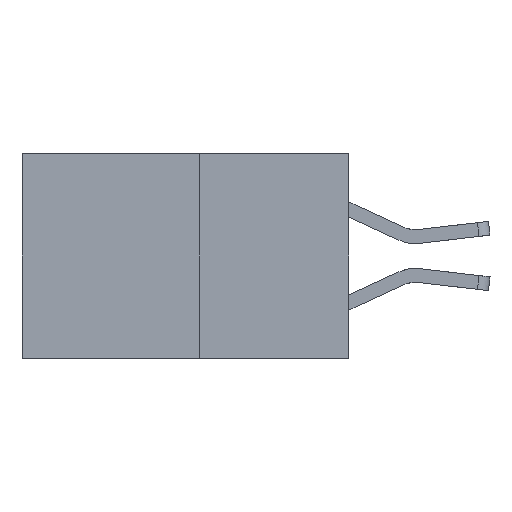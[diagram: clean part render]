
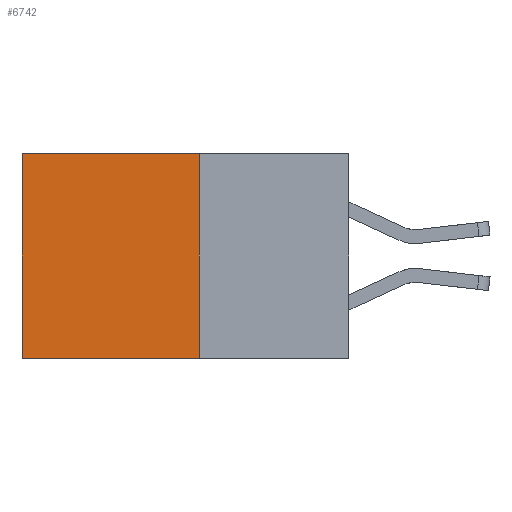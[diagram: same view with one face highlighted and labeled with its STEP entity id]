
A CAD part, left-side view. The second image highlights one B-rep face of the part: STEP entity #6742.
In plain terms, the highlighted planar face has unit normal (-1, 0, 0).
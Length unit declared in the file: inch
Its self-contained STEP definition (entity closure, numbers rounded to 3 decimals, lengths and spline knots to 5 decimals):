
#52 = ORIENTED_EDGE ( 'NONE', *, *, #1858, .T. ) ;
#1047 = VECTOR ( 'NONE', #1364, 39.37008 ) ;
#1349 = LINE ( 'NONE', #10455, #1047 ) ;
#1364 = DIRECTION ( 'NONE',  ( 0., 1., 0. ) ) ;
#1858 = EDGE_CURVE ( 'NONE', #4955, #6531, #1982, .T. ) ;
#1945 = LINE ( 'NONE', #10890, #11293 ) ;
#1982 = LINE ( 'NONE', #11210, #6603 ) ;
#2382 = ORIENTED_EDGE ( 'NONE', *, *, #6188, .F. ) ;
#2628 = PLANE ( 'NONE',  #7775 ) ;
#3532 = CARTESIAN_POINT ( 'NONE',  ( 0.277, 0.59, -0.37 ) ) ;
#3776 = VERTEX_POINT ( 'NONE', #3532 ) ;
#4144 = CARTESIAN_POINT ( 'NONE',  ( 0.277, 0.59, 0. ) ) ;
#4489 = CARTESIAN_POINT ( 'NONE',  ( 0.277, 0.27, -0.37 ) ) ;
#4505 = EDGE_CURVE ( 'NONE', #6531, #3776, #9742, .T. ) ;
#4569 = ORIENTED_EDGE ( 'NONE', *, *, #5871, .F. ) ;
#4955 = VERTEX_POINT ( 'NONE', #5926 ) ;
#5400 = DIRECTION ( 'NONE',  ( 1., 0., 0. ) ) ;
#5871 = EDGE_CURVE ( 'NONE', #10681, #3776, #1349, .T. ) ;
#5926 = CARTESIAN_POINT ( 'NONE',  ( 0.277, 0.27, 0. ) ) ;
#6188 = EDGE_CURVE ( 'NONE', #4955, #10681, #1945, .T. ) ;
#6531 = VERTEX_POINT ( 'NONE', #4144 ) ;
#6603 = VECTOR ( 'NONE', #11321, 39.37008 ) ;
#6690 = ORIENTED_EDGE ( 'NONE', *, *, #4505, .T. ) ;
#6742 = ADVANCED_FACE ( 'NONE', ( #9196 ), #2628, .F. ) ;
#6964 = CARTESIAN_POINT ( 'NONE',  ( 0.277, 0.27, -0.37 ) ) ;
#7775 = AXIS2_PLACEMENT_3D ( 'NONE', #4489, #5400, #11611 ) ;
#8327 = DIRECTION ( 'NONE',  ( 0., 0., -1. ) ) ;
#9196 = FACE_OUTER_BOUND ( 'NONE', #10832, .T. ) ;
#9742 = LINE ( 'NONE', #11450, #11726 ) ;
#10455 = CARTESIAN_POINT ( 'NONE',  ( 0.277, 0.27, -0.37 ) ) ;
#10681 = VERTEX_POINT ( 'NONE', #6964 ) ;
#10832 = EDGE_LOOP ( 'NONE', ( #6690, #4569, #2382, #52 ) ) ;
#10890 = CARTESIAN_POINT ( 'NONE',  ( 0.277, 0.27, -0.37 ) ) ;
#11210 = CARTESIAN_POINT ( 'NONE',  ( 0.277, 0.27, 0. ) ) ;
#11293 = VECTOR ( 'NONE', #8327, 39.37008 ) ;
#11321 = DIRECTION ( 'NONE',  ( 0., 1., 0. ) ) ;
#11450 = CARTESIAN_POINT ( 'NONE',  ( 0.277, 0.59, -0.37 ) ) ;
#11557 = DIRECTION ( 'NONE',  ( 0., 0., -1. ) ) ;
#11611 = DIRECTION ( 'NONE',  ( 0., 0., -1. ) ) ;
#11726 = VECTOR ( 'NONE', #11557, 39.37008 ) ;
